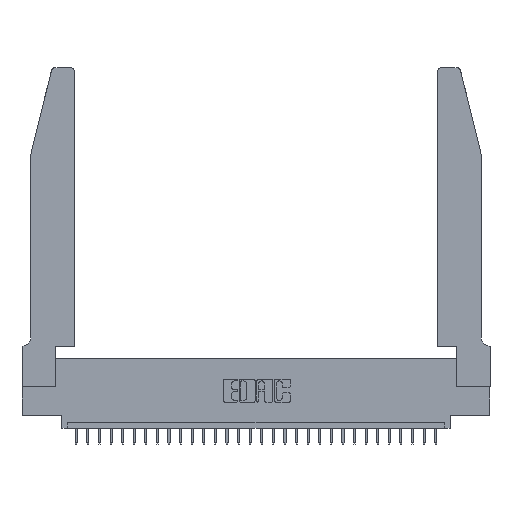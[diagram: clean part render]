
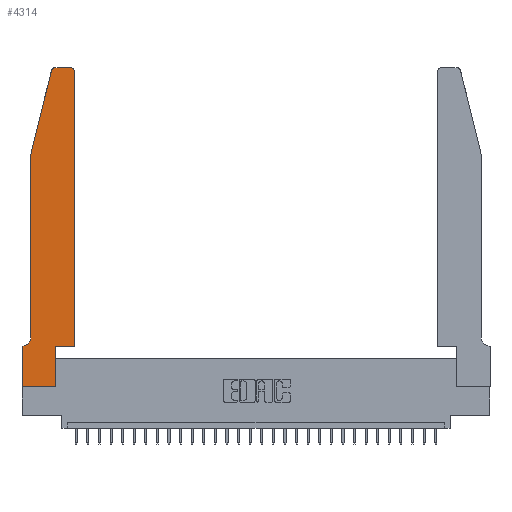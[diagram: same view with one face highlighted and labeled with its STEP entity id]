
A CAD part, top view. The second image highlights one B-rep face of the part: STEP entity #4314.
In plain terms, the highlighted planar face has unit normal (0, 0, 1).
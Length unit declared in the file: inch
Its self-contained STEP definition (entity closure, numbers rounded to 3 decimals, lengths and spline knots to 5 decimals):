
#201 = LINE ( 'NONE', #28338, #9450 ) ;
#1091 = VERTEX_POINT ( 'NONE', #5434 ) ;
#1137 = EDGE_CURVE ( 'NONE', #26112, #1091, #12530, .T. ) ;
#1308 = ORIENTED_EDGE ( 'NONE', *, *, #21409, .T. ) ;
#1472 = EDGE_CURVE ( 'NONE', #20917, #6663, #28928, .T. ) ;
#1560 = CARTESIAN_POINT ( 'NONE',  ( 0.284, 2.75, 0.37 ) ) ;
#4000 = ORIENTED_EDGE ( 'NONE', *, *, #5214, .T. ) ;
#4058 = LINE ( 'NONE', #8988, #29167 ) ;
#4314 = ADVANCED_FACE ( 'NONE', ( #16324 ), #21227, .T. ) ;
#5062 = EDGE_CURVE ( 'NONE', #10652, #23558, #4058, .T. ) ;
#5069 = CARTESIAN_POINT ( 'NONE',  ( 0., 0.35, 0.37 ) ) ;
#5091 = CARTESIAN_POINT ( 'NONE',  ( 0., 0., 0.37 ) ) ;
#5214 = EDGE_CURVE ( 'NONE', #6663, #29966, #201, .T. ) ;
#5239 = DIRECTION ( 'NONE',  ( 0., -1., 0. ) ) ;
#5363 = EDGE_CURVE ( 'NONE', #12094, #10652, #25716, .T. ) ;
#5395 = DIRECTION ( 'NONE',  ( 1., 0., 0. ) ) ;
#5416 = VECTOR ( 'NONE', #26961, 39.37008 ) ;
#5434 = CARTESIAN_POINT ( 'NONE',  ( 0.0755, 2., 0.37 ) ) ;
#6354 = CIRCLE ( 'NONE', #6859, 0.07 ) ;
#6663 = VERTEX_POINT ( 'NONE', #27328 ) ;
#6859 = AXIS2_PLACEMENT_3D ( 'NONE', #7738, #17126, #14815 ) ;
#6864 = LINE ( 'NONE', #16249, #17778 ) ;
#7146 = CARTESIAN_POINT ( 'NONE',  ( 0., 0.35, 0.37 ) ) ;
#7321 = CARTESIAN_POINT ( 'NONE',  ( 0.25487, 2.72718, 0.37 ) ) ;
#7706 = DIRECTION ( 'NONE',  ( 1., 0., 0. ) ) ;
#7738 = CARTESIAN_POINT ( 'NONE',  ( 0.0055, 0.42, 0.37 ) ) ;
#7784 = VERTEX_POINT ( 'NONE', #12022 ) ;
#8391 = VECTOR ( 'NONE', #5239, 39.37008 ) ;
#8493 = CARTESIAN_POINT ( 'NONE',  ( 0.4205, 2.72, 0.37 ) ) ;
#8850 = ORIENTED_EDGE ( 'NONE', *, *, #27969, .T. ) ;
#8988 = CARTESIAN_POINT ( 'NONE',  ( 0.2605, 2.75, 0.37 ) ) ;
#9390 = DIRECTION ( 'NONE',  ( 0., 0., 1. ) ) ;
#9450 = VECTOR ( 'NONE', #28489, 39.37008 ) ;
#9713 = CARTESIAN_POINT ( 'NONE',  ( 0.4505, 0.35, 0.37 ) ) ;
#9805 = ORIENTED_EDGE ( 'NONE', *, *, #17263, .T. ) ;
#10000 = AXIS2_PLACEMENT_3D ( 'NONE', #5069, #23821, #30302 ) ;
#10202 = DIRECTION ( 'NONE',  ( 1., 0., 0. ) ) ;
#10299 = LINE ( 'NONE', #26595, #20681 ) ;
#10652 = VERTEX_POINT ( 'NONE', #23119 ) ;
#12022 = CARTESIAN_POINT ( 'NONE',  ( 0.0755, 0.42, 0.37 ) ) ;
#12094 = VERTEX_POINT ( 'NONE', #12572 ) ;
#12335 = ORIENTED_EDGE ( 'NONE', *, *, #26763, .T. ) ;
#12530 = LINE ( 'NONE', #28812, #5416 ) ;
#12572 = CARTESIAN_POINT ( 'NONE',  ( 0.4505, 2.72, 0.37 ) ) ;
#14231 = DIRECTION ( 'NONE',  ( 0., -1., 0. ) ) ;
#14815 = DIRECTION ( 'NONE',  ( -1., 0., 0. ) ) ;
#14874 = ORIENTED_EDGE ( 'NONE', *, *, #23686, .T. ) ;
#15126 = LINE ( 'NONE', #19739, #22114 ) ;
#16249 = CARTESIAN_POINT ( 'NONE',  ( 0.0755, 2., 0.37 ) ) ;
#16324 = FACE_OUTER_BOUND ( 'NONE', #23382, .T. ) ;
#16393 = CARTESIAN_POINT ( 'NONE',  ( 0.0055, 0.35, 0.37 ) ) ;
#16508 = AXIS2_PLACEMENT_3D ( 'NONE', #25834, #9390, #7706 ) ;
#17126 = DIRECTION ( 'NONE',  ( 0., 0., -1. ) ) ;
#17263 = EDGE_CURVE ( 'NONE', #28476, #12094, #10299, .T. ) ;
#17778 = VECTOR ( 'NONE', #14231, 39.37008 ) ;
#18131 = ORIENTED_EDGE ( 'NONE', *, *, #1137, .T. ) ;
#18480 = VERTEX_POINT ( 'NONE', #21070 ) ;
#19264 = EDGE_CURVE ( 'NONE', #1091, #7784, #6864, .T. ) ;
#19739 = CARTESIAN_POINT ( 'NONE',  ( 0.0755, 0.35, 0.37 ) ) ;
#19881 = DIRECTION ( 'NONE',  ( 0., 0., 1. ) ) ;
#20333 = AXIS2_PLACEMENT_3D ( 'NONE', #8493, #19881, #10202 ) ;
#20681 = VECTOR ( 'NONE', #28597, 39.37008 ) ;
#20805 = CARTESIAN_POINT ( 'NONE',  ( 0.2865, 0., 0.37 ) ) ;
#20917 = VERTEX_POINT ( 'NONE', #7146 ) ;
#20960 = ORIENTED_EDGE ( 'NONE', *, *, #1472, .T. ) ;
#21070 = CARTESIAN_POINT ( 'NONE',  ( 0.2865, 0.35, 0.37 ) ) ;
#21227 = PLANE ( 'NONE',  #10000 ) ;
#21409 = EDGE_CURVE ( 'NONE', #18480, #28476, #23991, .T. ) ;
#21835 = CARTESIAN_POINT ( 'NONE',  ( 0.2865, 0.35, 0.37 ) ) ;
#21882 = DIRECTION ( 'NONE',  ( -1., 0., 0. ) ) ;
#21968 = EDGE_CURVE ( 'NONE', #29966, #18480, #26139, .T. ) ;
#22114 = VECTOR ( 'NONE', #21882, 39.37008 ) ;
#22811 = DIRECTION ( 'NONE',  ( -1., 0., 0. ) ) ;
#23119 = CARTESIAN_POINT ( 'NONE',  ( 0.4205, 2.75, 0.37 ) ) ;
#23382 = EDGE_LOOP ( 'NONE', ( #25768, #14874, #18131, #23864, #12335, #8850, #20960, #4000, #27838, #1308, #9805, #24630 ) ) ;
#23558 = VERTEX_POINT ( 'NONE', #1560 ) ;
#23686 = EDGE_CURVE ( 'NONE', #23558, #26112, #29768, .T. ) ;
#23704 = VECTOR ( 'NONE', #29216, 39.37008 ) ;
#23821 = DIRECTION ( 'NONE',  ( 0., 0., 1. ) ) ;
#23864 = ORIENTED_EDGE ( 'NONE', *, *, #19264, .T. ) ;
#23991 = LINE ( 'NONE', #9713, #28622 ) ;
#24630 = ORIENTED_EDGE ( 'NONE', *, *, #5363, .T. ) ;
#25716 = CIRCLE ( 'NONE', #20333, 0.03 ) ;
#25768 = ORIENTED_EDGE ( 'NONE', *, *, #5062, .T. ) ;
#25834 = CARTESIAN_POINT ( 'NONE',  ( 0.284, 2.72, 0.37 ) ) ;
#26112 = VERTEX_POINT ( 'NONE', #7321 ) ;
#26139 = LINE ( 'NONE', #21835, #23704 ) ;
#26595 = CARTESIAN_POINT ( 'NONE',  ( 0.4505, 0.35, 0.37 ) ) ;
#26763 = EDGE_CURVE ( 'NONE', #7784, #29785, #6354, .T. ) ;
#26961 = DIRECTION ( 'NONE',  ( -0.239, -0.971, 0. ) ) ;
#27328 = CARTESIAN_POINT ( 'NONE',  ( 0., 0., 0.37 ) ) ;
#27838 = ORIENTED_EDGE ( 'NONE', *, *, #21968, .T. ) ;
#27969 = EDGE_CURVE ( 'NONE', #29785, #20917, #15126, .T. ) ;
#28338 = CARTESIAN_POINT ( 'NONE',  ( 0., 0., 0.37 ) ) ;
#28476 = VERTEX_POINT ( 'NONE', #29228 ) ;
#28489 = DIRECTION ( 'NONE',  ( 1., 0., 0. ) ) ;
#28597 = DIRECTION ( 'NONE',  ( 0., 1., 0. ) ) ;
#28622 = VECTOR ( 'NONE', #5395, 39.37008 ) ;
#28812 = CARTESIAN_POINT ( 'NONE',  ( 0.0755, 2., 0.37 ) ) ;
#28928 = LINE ( 'NONE', #5091, #8391 ) ;
#29167 = VECTOR ( 'NONE', #22811, 39.37008 ) ;
#29216 = DIRECTION ( 'NONE',  ( 0., 1., 0. ) ) ;
#29228 = CARTESIAN_POINT ( 'NONE',  ( 0.4505, 0.35, 0.37 ) ) ;
#29768 = CIRCLE ( 'NONE', #16508, 0.03 ) ;
#29785 = VERTEX_POINT ( 'NONE', #16393 ) ;
#29966 = VERTEX_POINT ( 'NONE', #20805 ) ;
#30302 = DIRECTION ( 'NONE',  ( 1., 0., 0. ) ) ;
